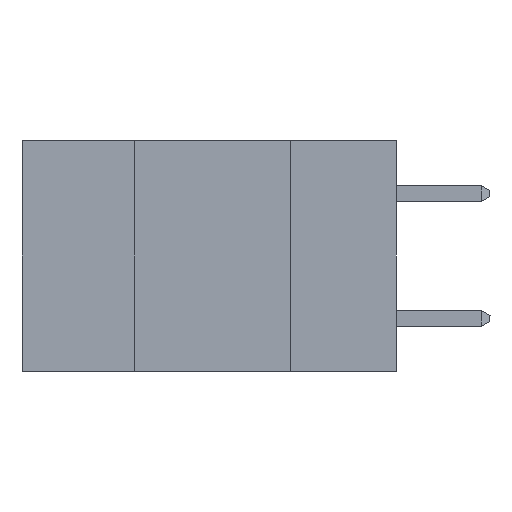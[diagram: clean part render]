
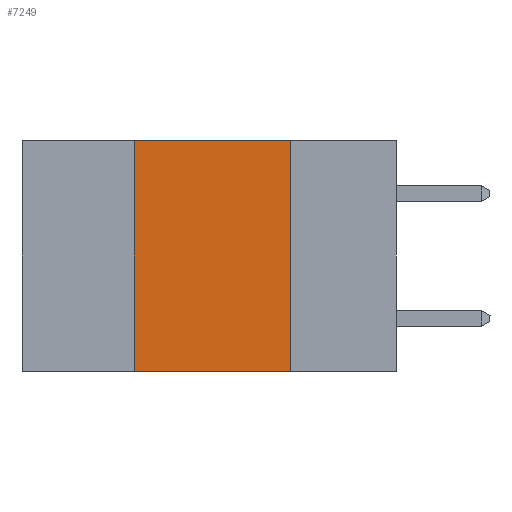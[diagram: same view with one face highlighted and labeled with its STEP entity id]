
A CAD part, left-side view. The second image highlights one B-rep face of the part: STEP entity #7249.
In plain terms, the highlighted planar face has unit normal (-1, 0, 0).
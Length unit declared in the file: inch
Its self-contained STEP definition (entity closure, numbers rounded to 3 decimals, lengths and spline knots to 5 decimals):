
#360 = EDGE_LOOP ( 'NONE', ( #466, #8745, #7137, #16572 ) ) ;
#466 = ORIENTED_EDGE ( 'NONE', *, *, #6071, .F. ) ;
#1401 = DIRECTION ( 'NONE',  ( 0., -1., 0. ) ) ;
#2291 = CARTESIAN_POINT ( 'NONE',  ( 0., 0.42, -0.37 ) ) ;
#3364 = VECTOR ( 'NONE', #12532, 39.37008 ) ;
#3994 = VERTEX_POINT ( 'NONE', #5091 ) ;
#4348 = EDGE_CURVE ( 'NONE', #4696, #3994, #13866, .T. ) ;
#4529 = VECTOR ( 'NONE', #14758, 39.37008 ) ;
#4696 = VERTEX_POINT ( 'NONE', #2291 ) ;
#4968 = LINE ( 'NONE', #17484, #4529 ) ;
#5091 = CARTESIAN_POINT ( 'NONE',  ( 0., 0.17, -0.37 ) ) ;
#5922 = FACE_OUTER_BOUND ( 'NONE', #360, .T. ) ;
#6071 = EDGE_CURVE ( 'NONE', #16028, #3994, #10773, .T. ) ;
#6431 = VECTOR ( 'NONE', #11883, 39.37008 ) ;
#7137 = ORIENTED_EDGE ( 'NONE', *, *, #16961, .F. ) ;
#7249 = ADVANCED_FACE ( 'NONE', ( #5922 ), #12514, .F. ) ;
#8745 = ORIENTED_EDGE ( 'NONE', *, *, #14253, .F. ) ;
#9212 = CARTESIAN_POINT ( 'NONE',  ( 0., 0.42, 0. ) ) ;
#10773 = LINE ( 'NONE', #11237, #3364 ) ;
#11237 = CARTESIAN_POINT ( 'NONE',  ( 0., 0.17, -0.37 ) ) ;
#11765 = DIRECTION ( 'NONE',  ( 0., 0., -1. ) ) ;
#11883 = DIRECTION ( 'NONE',  ( 0., -1., 0. ) ) ;
#11977 = DIRECTION ( 'NONE',  ( 1., 0., 0. ) ) ;
#12317 = CARTESIAN_POINT ( 'NONE',  ( 0., 0.6, 0. ) ) ;
#12514 = PLANE ( 'NONE',  #14535 ) ;
#12532 = DIRECTION ( 'NONE',  ( 0., 0., -1. ) ) ;
#12757 = CARTESIAN_POINT ( 'NONE',  ( 0., 0.6, -0.37 ) ) ;
#13866 = LINE ( 'NONE', #12757, #6431 ) ;
#14002 = VERTEX_POINT ( 'NONE', #9212 ) ;
#14244 = CARTESIAN_POINT ( 'NONE',  ( 0., 0.17, 0. ) ) ;
#14253 = EDGE_CURVE ( 'NONE', #14002, #16028, #15906, .T. ) ;
#14535 = AXIS2_PLACEMENT_3D ( 'NONE', #12317, #11977, #11765 ) ;
#14758 = DIRECTION ( 'NONE',  ( 0., 0., 1. ) ) ;
#15303 = CARTESIAN_POINT ( 'NONE',  ( 0., 0.6, 0. ) ) ;
#15478 = VECTOR ( 'NONE', #1401, 39.37008 ) ;
#15906 = LINE ( 'NONE', #15303, #15478 ) ;
#16028 = VERTEX_POINT ( 'NONE', #14244 ) ;
#16572 = ORIENTED_EDGE ( 'NONE', *, *, #4348, .T. ) ;
#16961 = EDGE_CURVE ( 'NONE', #4696, #14002, #4968, .T. ) ;
#17484 = CARTESIAN_POINT ( 'NONE',  ( 0., 0.42, -0.37 ) ) ;
